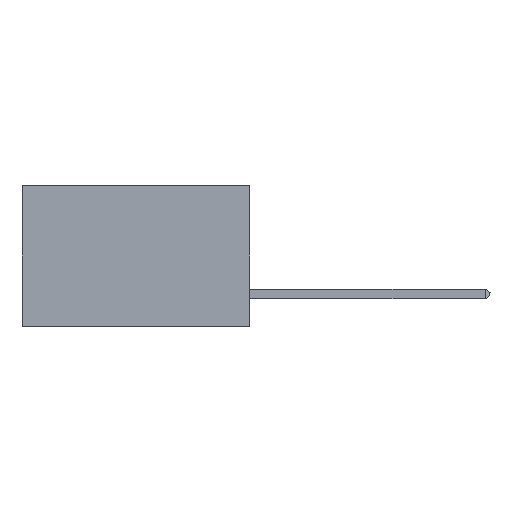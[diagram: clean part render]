
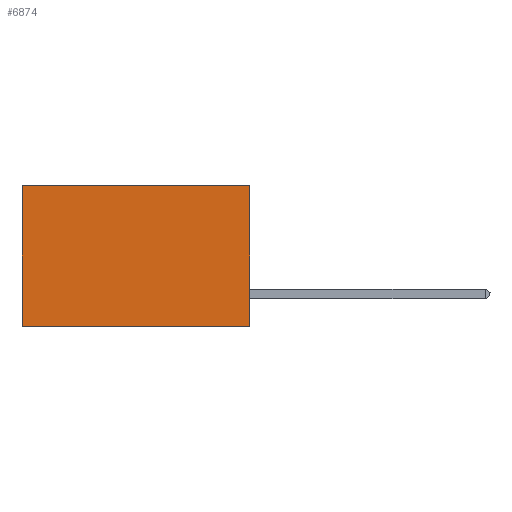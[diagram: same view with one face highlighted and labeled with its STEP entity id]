
A CAD part, left-side view. The second image highlights one B-rep face of the part: STEP entity #6874.
In plain terms, the highlighted planar face has unit normal (-1, 0, 0).
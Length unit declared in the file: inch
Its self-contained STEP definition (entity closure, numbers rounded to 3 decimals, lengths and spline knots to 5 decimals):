
#5607 = VECTOR ( 'NONE', #21275, 39.37008 ) ;
#5780 = DIRECTION ( 'NONE',  ( 0., 0., -1. ) ) ;
#6323 = EDGE_CURVE ( 'NONE', #14612, #28513, #11818, .T. ) ;
#6874 = ADVANCED_FACE ( 'NONE', ( #30082 ), #43972, .F. ) ;
#6899 = DIRECTION ( 'NONE',  ( 0., 1., 0. ) ) ;
#11193 = LINE ( 'NONE', #27658, #16597 ) ;
#11818 = LINE ( 'NONE', #15508, #33847 ) ;
#11885 = DIRECTION ( 'NONE',  ( 0., 1., 0. ) ) ;
#13747 = VERTEX_POINT ( 'NONE', #42642 ) ;
#14612 = VERTEX_POINT ( 'NONE', #19172 ) ;
#15508 = CARTESIAN_POINT ( 'NONE',  ( 0.2875, 0., -0.37 ) ) ;
#16475 = VECTOR ( 'NONE', #27304, 39.37008 ) ;
#16597 = VECTOR ( 'NONE', #6899, 39.37008 ) ;
#19172 = CARTESIAN_POINT ( 'NONE',  ( 0.2875, 0., -0.37 ) ) ;
#21252 = EDGE_LOOP ( 'NONE', ( #37145, #27474, #27386, #43698 ) ) ;
#21275 = DIRECTION ( 'NONE',  ( 0., 0., -1. ) ) ;
#21385 = EDGE_CURVE ( 'NONE', #31377, #28513, #25978, .T. ) ;
#25978 = LINE ( 'NONE', #38252, #5607 ) ;
#27200 = LINE ( 'NONE', #37798, #16475 ) ;
#27304 = DIRECTION ( 'NONE',  ( 0., 0., -1. ) ) ;
#27386 = ORIENTED_EDGE ( 'NONE', *, *, #43561, .F. ) ;
#27474 = ORIENTED_EDGE ( 'NONE', *, *, #6323, .F. ) ;
#27658 = CARTESIAN_POINT ( 'NONE',  ( 0.2875, 0., 0. ) ) ;
#28513 = VERTEX_POINT ( 'NONE', #42287 ) ;
#30082 = FACE_OUTER_BOUND ( 'NONE', #21252, .T. ) ;
#30353 = CARTESIAN_POINT ( 'NONE',  ( 0.2875, 0., 0. ) ) ;
#31377 = VERTEX_POINT ( 'NONE', #34266 ) ;
#33847 = VECTOR ( 'NONE', #11885, 39.37008 ) ;
#34266 = CARTESIAN_POINT ( 'NONE',  ( 0.2875, 0.6, 0. ) ) ;
#34361 = AXIS2_PLACEMENT_3D ( 'NONE', #30353, #36527, #5780 ) ;
#36527 = DIRECTION ( 'NONE',  ( 1., 0., 0. ) ) ;
#37145 = ORIENTED_EDGE ( 'NONE', *, *, #21385, .T. ) ;
#37798 = CARTESIAN_POINT ( 'NONE',  ( 0.2875, 0., 0. ) ) ;
#38252 = CARTESIAN_POINT ( 'NONE',  ( 0.2875, 0.6, 0. ) ) ;
#42287 = CARTESIAN_POINT ( 'NONE',  ( 0.2875, 0.6, -0.37 ) ) ;
#42357 = EDGE_CURVE ( 'NONE', #13747, #31377, #11193, .T. ) ;
#42642 = CARTESIAN_POINT ( 'NONE',  ( 0.2875, 0., 0. ) ) ;
#43561 = EDGE_CURVE ( 'NONE', #13747, #14612, #27200, .T. ) ;
#43698 = ORIENTED_EDGE ( 'NONE', *, *, #42357, .T. ) ;
#43972 = PLANE ( 'NONE',  #34361 ) ;
